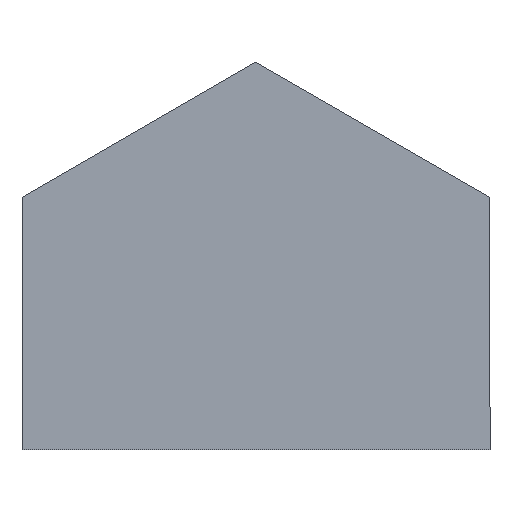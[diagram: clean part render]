
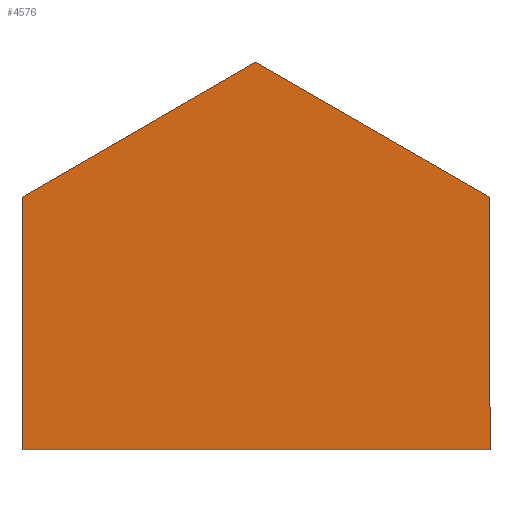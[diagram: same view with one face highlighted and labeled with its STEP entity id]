
A CAD part, left-side view. The second image highlights one B-rep face of the part: STEP entity #4576.
In plain terms, the highlighted planar face has unit normal (-1, 0, 0).
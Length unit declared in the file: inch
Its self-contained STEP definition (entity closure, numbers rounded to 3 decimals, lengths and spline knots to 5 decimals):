
#152 = EDGE_CURVE ( 'NONE', #2218, #2925, #4848, .T. ) ;
#281 = DIRECTION ( 'NONE',  ( 0., 1., 0. ) ) ;
#339 = ORIENTED_EDGE ( 'NONE', *, *, #2383, .T. ) ;
#679 = CARTESIAN_POINT ( 'NONE',  ( -1.05656, 0.76964, -0.70913 ) ) ;
#773 = LINE ( 'NONE', #3773, #1948 ) ;
#1202 = CARTESIAN_POINT ( 'NONE',  ( -1.05656, 0.98464, -0.33673 ) ) ;
#1286 = CARTESIAN_POINT ( 'NONE',  ( -1.05656, 1.19964, -0.46086 ) ) ;
#1322 = LINE ( 'NONE', #2953, #4124 ) ;
#1792 = AXIS2_PLACEMENT_3D ( 'NONE', #5218, #3846, #4305 ) ;
#1948 = VECTOR ( 'NONE', #4235, 39.37008 ) ;
#2120 = VERTEX_POINT ( 'NONE', #2924 ) ;
#2144 = LINE ( 'NONE', #3312, #5038 ) ;
#2218 = VERTEX_POINT ( 'NONE', #5543 ) ;
#2230 = VECTOR ( 'NONE', #4259, 39.37008 ) ;
#2383 = EDGE_CURVE ( 'NONE', #4755, #2120, #1322, .T. ) ;
#2807 = EDGE_CURVE ( 'NONE', #3663, #4755, #4481, .T. ) ;
#2821 = CARTESIAN_POINT ( 'NONE',  ( -1.05656, 0.76964, -0.46086 ) ) ;
#2924 = CARTESIAN_POINT ( 'NONE',  ( -1.05656, 1.19964, -0.6931 ) ) ;
#2925 = VERTEX_POINT ( 'NONE', #2821 ) ;
#2953 = CARTESIAN_POINT ( 'NONE',  ( -1.05656, 1.19964, -0.46086 ) ) ;
#3199 = EDGE_CURVE ( 'NONE', #2218, #2120, #2144, .T. ) ;
#3271 = VECTOR ( 'NONE', #3585, 39.37008 ) ;
#3312 = CARTESIAN_POINT ( 'NONE',  ( -1.05656, 0.98464, -0.6931 ) ) ;
#3392 = PLANE ( 'NONE',  #1792 ) ;
#3575 = EDGE_CURVE ( 'NONE', #2925, #3663, #773, .T. ) ;
#3585 = DIRECTION ( 'NONE',  ( 0., 0.866, -0.5 ) ) ;
#3663 = VERTEX_POINT ( 'NONE', #1202 ) ;
#3773 = CARTESIAN_POINT ( 'NONE',  ( -1.05656, 0.76964, -0.46086 ) ) ;
#3846 = DIRECTION ( 'NONE',  ( -1., 0., 0. ) ) ;
#3876 = ORIENTED_EDGE ( 'NONE', *, *, #3199, .F. ) ;
#3885 = DIRECTION ( 'NONE',  ( 0., 0., -1. ) ) ;
#3887 = ORIENTED_EDGE ( 'NONE', *, *, #152, .T. ) ;
#4124 = VECTOR ( 'NONE', #3885, 39.37008 ) ;
#4235 = DIRECTION ( 'NONE',  ( 0., 0.866, 0.5 ) ) ;
#4259 = DIRECTION ( 'NONE',  ( 0., 0., 1. ) ) ;
#4305 = DIRECTION ( 'NONE',  ( 0., 0., 1. ) ) ;
#4312 = EDGE_LOOP ( 'NONE', ( #3876, #3887, #5710, #4727, #339 ) ) ;
#4481 = LINE ( 'NONE', #4503, #3271 ) ;
#4503 = CARTESIAN_POINT ( 'NONE',  ( -1.05656, 0.98464, -0.33673 ) ) ;
#4576 = ADVANCED_FACE ( 'NONE', ( #5103 ), #3392, .T. ) ;
#4727 = ORIENTED_EDGE ( 'NONE', *, *, #2807, .T. ) ;
#4755 = VERTEX_POINT ( 'NONE', #1286 ) ;
#4848 = LINE ( 'NONE', #679, #2230 ) ;
#5038 = VECTOR ( 'NONE', #281, 39.37008 ) ;
#5103 = FACE_OUTER_BOUND ( 'NONE', #4312, .T. ) ;
#5218 = CARTESIAN_POINT ( 'NONE',  ( -1.05656, 0.98464, -0.585 ) ) ;
#5543 = CARTESIAN_POINT ( 'NONE',  ( -1.05656, 0.76964, -0.6931 ) ) ;
#5710 = ORIENTED_EDGE ( 'NONE', *, *, #3575, .T. ) ;
